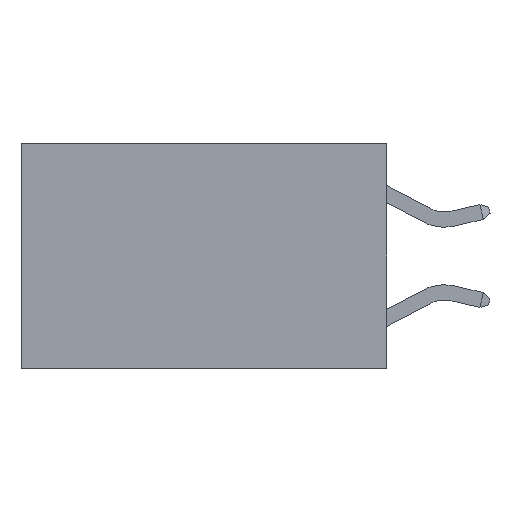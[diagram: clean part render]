
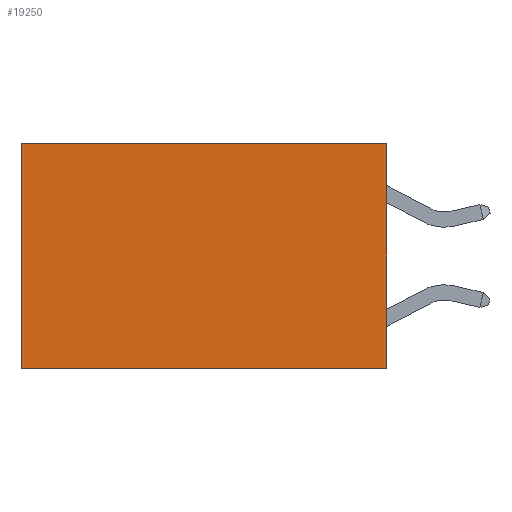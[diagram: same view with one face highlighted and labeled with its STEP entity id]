
A CAD part, left-side view. The second image highlights one B-rep face of the part: STEP entity #19250.
In plain terms, the highlighted planar face has unit normal (-1, 0, 0).
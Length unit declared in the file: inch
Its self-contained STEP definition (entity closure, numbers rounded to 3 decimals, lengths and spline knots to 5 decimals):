
#183 = PLANE ( 'NONE',  #11043 ) ;
#479 = EDGE_LOOP ( 'NONE', ( #19068, #11915, #4303, #17805 ) ) ;
#494 = FACE_OUTER_BOUND ( 'NONE', #479, .T. ) ;
#1127 = CARTESIAN_POINT ( 'NONE',  ( 0.2625, 0., 0. ) ) ;
#1140 = VECTOR ( 'NONE', #20837, 39.37008 ) ;
#1367 = DIRECTION ( 'NONE',  ( 0., 0., -1. ) ) ;
#1621 = CARTESIAN_POINT ( 'NONE',  ( 0.2625, 0., -0.37 ) ) ;
#3461 = EDGE_CURVE ( 'NONE', #9824, #7095, #14166, .T. ) ;
#3508 = DIRECTION ( 'NONE',  ( 1., 0., 0. ) ) ;
#4032 = CARTESIAN_POINT ( 'NONE',  ( 0.2625, 0.6, -0.37 ) ) ;
#4303 = ORIENTED_EDGE ( 'NONE', *, *, #16890, .F. ) ;
#4340 = VERTEX_POINT ( 'NONE', #4362 ) ;
#4362 = CARTESIAN_POINT ( 'NONE',  ( 0.2625, 0., 0. ) ) ;
#7095 = VERTEX_POINT ( 'NONE', #4032 ) ;
#8172 = EDGE_CURVE ( 'NONE', #4340, #14707, #10706, .T. ) ;
#9824 = VERTEX_POINT ( 'NONE', #1621 ) ;
#10706 = LINE ( 'NONE', #1127, #19396 ) ;
#11043 = AXIS2_PLACEMENT_3D ( 'NONE', #19773, #3508, #14929 ) ;
#11156 = CARTESIAN_POINT ( 'NONE',  ( 0.2625, 0., 0. ) ) ;
#11915 = ORIENTED_EDGE ( 'NONE', *, *, #3461, .F. ) ;
#12328 = VECTOR ( 'NONE', #12780, 39.37008 ) ;
#12511 = DIRECTION ( 'NONE',  ( 0., 1., 0. ) ) ;
#12689 = CARTESIAN_POINT ( 'NONE',  ( 0.2625, 0., -0.37 ) ) ;
#12780 = DIRECTION ( 'NONE',  ( 0., 0., -1. ) ) ;
#13360 = LINE ( 'NONE', #11156, #12328 ) ;
#14166 = LINE ( 'NONE', #12689, #1140 ) ;
#14425 = CARTESIAN_POINT ( 'NONE',  ( 0.2625, 0.6, 0. ) ) ;
#14548 = LINE ( 'NONE', #14425, #18368 ) ;
#14707 = VERTEX_POINT ( 'NONE', #20216 ) ;
#14929 = DIRECTION ( 'NONE',  ( 0., 0., -1. ) ) ;
#16890 = EDGE_CURVE ( 'NONE', #4340, #9824, #13360, .T. ) ;
#17805 = ORIENTED_EDGE ( 'NONE', *, *, #8172, .T. ) ;
#18368 = VECTOR ( 'NONE', #1367, 39.37008 ) ;
#19068 = ORIENTED_EDGE ( 'NONE', *, *, #19192, .T. ) ;
#19192 = EDGE_CURVE ( 'NONE', #14707, #7095, #14548, .T. ) ;
#19250 = ADVANCED_FACE ( 'NONE', ( #494 ), #183, .F. ) ;
#19396 = VECTOR ( 'NONE', #12511, 39.37008 ) ;
#19773 = CARTESIAN_POINT ( 'NONE',  ( 0.2625, 0., 0. ) ) ;
#20216 = CARTESIAN_POINT ( 'NONE',  ( 0.2625, 0.6, 0. ) ) ;
#20837 = DIRECTION ( 'NONE',  ( 0., 1., 0. ) ) ;
